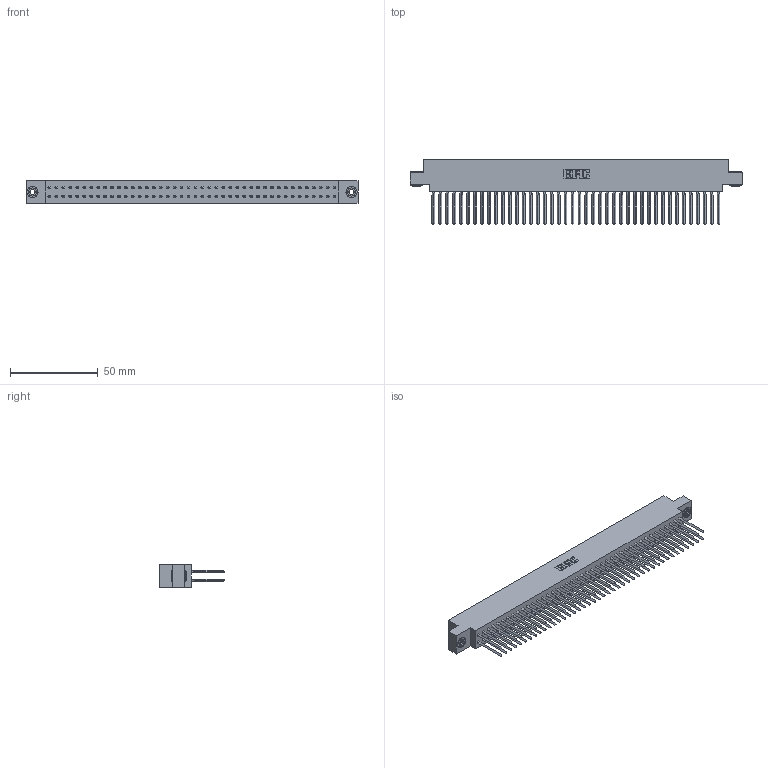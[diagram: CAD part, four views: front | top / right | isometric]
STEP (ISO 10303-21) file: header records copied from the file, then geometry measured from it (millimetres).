
FILE_DESCRIPTION (( 'STEP AP203' ), '1' );
FILE_NAME ('317-084-542-803.STEP', '2020-02-28T10:09:12', ( '' ), ( '' ), 'SwSTEP 2.0', 'SolidWorks 2016', '' );
FILE_SCHEMA (( 'CONFIG_CONTROL_DESIGN' ));
Length unit declared in the file: inch
Products named in the file (4): 317 Part_.156 Dia - TH; 317-084-542-803; 317-290-003_542; 345-250-002_345-250-002-102
Assembly tree (87 placements, depth 2):
  317-084-542-803
    317 Part_.156 Dia - TH
    317-290-003_542  x84
    345-250-002_345-250-002-102  x2
Bounding box: 189.13 x 37.34 x 12.7 mm (x, y, z)
Volume: 30988.5 mm3; surface area: 43308.6 mm2
Topology: 87 solids, 87 shells, 4928 faces, 13791 edges, 8798 vertices
Faces by surface type: plane 3932, cylinder 652, bspline 336, cone 8
Entity records: 60378 total; most frequent: CARTESIAN_POINT 10752, ORIENTED_EDGE 10408, DIRECTION 8794, EDGE_CURVE 5204, LINE 5010, VECTOR 5010, VERTEX_POINT 3462, AXIS2_PLACEMENT_3D 1892
